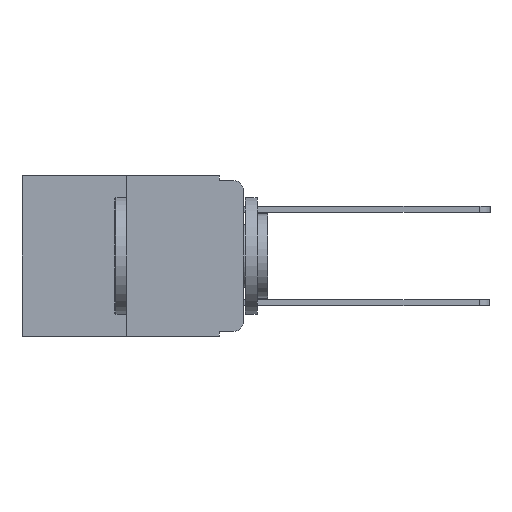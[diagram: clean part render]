
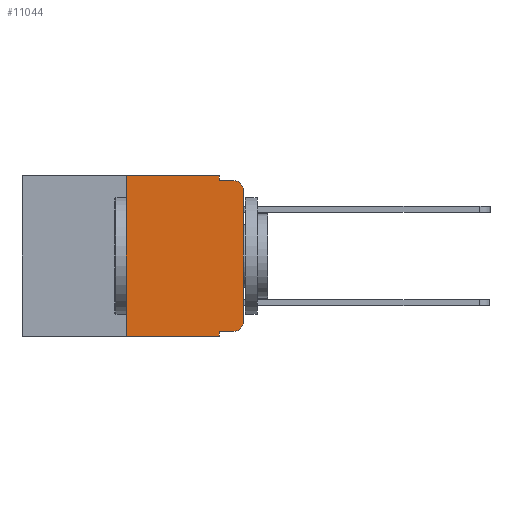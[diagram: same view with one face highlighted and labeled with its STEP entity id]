
A CAD part, left-side view. The second image highlights one B-rep face of the part: STEP entity #11044.
In plain terms, the highlighted planar face has unit normal (-1, 0, 0).
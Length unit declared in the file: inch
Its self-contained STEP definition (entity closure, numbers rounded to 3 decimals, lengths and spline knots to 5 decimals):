
#227 = VERTEX_POINT ( 'NONE', #5715 ) ;
#491 = ORIENTED_EDGE ( 'NONE', *, *, #11624, .F. ) ;
#746 = EDGE_CURVE ( 'NONE', #3006, #7960, #10381, .T. ) ;
#1089 = CARTESIAN_POINT ( 'NONE',  ( 0., 0., 0. ) ) ;
#1142 = VECTOR ( 'NONE', #10765, 39.37008 ) ;
#1330 = VECTOR ( 'NONE', #1624, 39.37008 ) ;
#1410 = CARTESIAN_POINT ( 'NONE',  ( 0., 0.25, -0.343 ) ) ;
#1515 = VECTOR ( 'NONE', #7484, 39.37008 ) ;
#1612 = LINE ( 'NONE', #1089, #14102 ) ;
#1624 = DIRECTION ( 'NONE',  ( 0., 0., -1. ) ) ;
#1700 = LINE ( 'NONE', #18387, #1142 ) ;
#1743 = DIRECTION ( 'NONE',  ( -1., 0., 0. ) ) ;
#2067 = AXIS2_PLACEMENT_3D ( 'NONE', #5316, #17886, #8572 ) ;
#2700 = ORIENTED_EDGE ( 'NONE', *, *, #9438, .T. ) ;
#2933 = DIRECTION ( 'NONE',  ( 0., 0., 1. ) ) ;
#3006 = VERTEX_POINT ( 'NONE', #1410 ) ;
#3287 = VERTEX_POINT ( 'NONE', #15945 ) ;
#3361 = DIRECTION ( 'NONE',  ( 0., -1., 0. ) ) ;
#3600 = CARTESIAN_POINT ( 'NONE',  ( 0., 0.02, -0.03 ) ) ;
#4095 = CARTESIAN_POINT ( 'NONE',  ( 0., 0.051, 0. ) ) ;
#4788 = ORIENTED_EDGE ( 'NONE', *, *, #15676, .T. ) ;
#5189 = CARTESIAN_POINT ( 'NONE',  ( 0., 0.02, -0.01 ) ) ;
#5312 = DIRECTION ( 'NONE',  ( 0., 0., -1. ) ) ;
#5316 = CARTESIAN_POINT ( 'NONE',  ( 0., 0.473, 0. ) ) ;
#5622 = ORIENTED_EDGE ( 'NONE', *, *, #10556, .T. ) ;
#5715 = CARTESIAN_POINT ( 'NONE',  ( 0., 0., -0.03 ) ) ;
#5943 = AXIS2_PLACEMENT_3D ( 'NONE', #3600, #14831, #5312 ) ;
#6291 = CARTESIAN_POINT ( 'NONE',  ( 0., 0.25, 0. ) ) ;
#6614 = CARTESIAN_POINT ( 'NONE',  ( 0., 0.051, 0. ) ) ;
#6912 = PLANE ( 'NONE',  #2067 ) ;
#7179 = CIRCLE ( 'NONE', #16317, 0.02 ) ;
#7484 = DIRECTION ( 'NONE',  ( 0., -1., 0. ) ) ;
#7960 = VERTEX_POINT ( 'NONE', #11419 ) ;
#8572 = DIRECTION ( 'NONE',  ( 0., 0., -1. ) ) ;
#8763 = CARTESIAN_POINT ( 'NONE',  ( 0., 0.02, -0.333 ) ) ;
#9198 = VERTEX_POINT ( 'NONE', #18639 ) ;
#9293 = CARTESIAN_POINT ( 'NONE',  ( 0., 0.051, -0.333 ) ) ;
#9438 = EDGE_CURVE ( 'NONE', #19296, #18883, #7179, .T. ) ;
#10018 = LINE ( 'NONE', #13117, #17720 ) ;
#10020 = EDGE_CURVE ( 'NONE', #3287, #9198, #10018, .T. ) ;
#10178 = ORIENTED_EDGE ( 'NONE', *, *, #14682, .F. ) ;
#10381 = LINE ( 'NONE', #16709, #1515 ) ;
#10556 = EDGE_CURVE ( 'NONE', #10694, #19296, #17216, .T. ) ;
#10694 = VERTEX_POINT ( 'NONE', #9293 ) ;
#10765 = DIRECTION ( 'NONE',  ( 0., -1., 0. ) ) ;
#11044 = ADVANCED_FACE ( 'NONE', ( #12233 ), #6912, .F. ) ;
#11165 = VECTOR ( 'NONE', #15243, 39.37008 ) ;
#11374 = LINE ( 'NONE', #6291, #18998 ) ;
#11419 = CARTESIAN_POINT ( 'NONE',  ( 0., 0.051, -0.343 ) ) ;
#11617 = EDGE_LOOP ( 'NONE', ( #13603, #4788, #10178, #12183, #13861, #17882, #20269, #491, #5622, #2700 ) ) ;
#11624 = EDGE_CURVE ( 'NONE', #10694, #7960, #17895, .T. ) ;
#11640 = CARTESIAN_POINT ( 'NONE',  ( 0., 0.02, -0.313 ) ) ;
#12183 = ORIENTED_EDGE ( 'NONE', *, *, #13694, .F. ) ;
#12233 = FACE_OUTER_BOUND ( 'NONE', #11617, .T. ) ;
#12241 = DIRECTION ( 'NONE',  ( 0., 0., -1. ) ) ;
#12547 = LINE ( 'NONE', #4095, #20148 ) ;
#12654 = EDGE_CURVE ( 'NONE', #3006, #3287, #11374, .T. ) ;
#13117 = CARTESIAN_POINT ( 'NONE',  ( 0., 0.473, 0. ) ) ;
#13208 = DIRECTION ( 'NONE',  ( 0., 0., -1. ) ) ;
#13603 = ORIENTED_EDGE ( 'NONE', *, *, #16724, .T. ) ;
#13694 = EDGE_CURVE ( 'NONE', #9198, #15691, #12547, .T. ) ;
#13861 = ORIENTED_EDGE ( 'NONE', *, *, #10020, .F. ) ;
#14102 = VECTOR ( 'NONE', #17198, 39.37008 ) ;
#14682 = EDGE_CURVE ( 'NONE', #15691, #19795, #1700, .T. ) ;
#14831 = DIRECTION ( 'NONE',  ( -1., 0., 0. ) ) ;
#15181 = CARTESIAN_POINT ( 'NONE',  ( 0., 0.051, -0.333 ) ) ;
#15243 = DIRECTION ( 'NONE',  ( 0., -1., 0. ) ) ;
#15676 = EDGE_CURVE ( 'NONE', #227, #19795, #17186, .T. ) ;
#15691 = VERTEX_POINT ( 'NONE', #16352 ) ;
#15945 = CARTESIAN_POINT ( 'NONE',  ( 0., 0.25, 0. ) ) ;
#16317 = AXIS2_PLACEMENT_3D ( 'NONE', #11640, #1743, #13208 ) ;
#16352 = CARTESIAN_POINT ( 'NONE',  ( 0., 0.051, -0.01 ) ) ;
#16709 = CARTESIAN_POINT ( 'NONE',  ( 0., 0.473, -0.343 ) ) ;
#16724 = EDGE_CURVE ( 'NONE', #18883, #227, #1612, .T. ) ;
#17186 = CIRCLE ( 'NONE', #5943, 0.02 ) ;
#17198 = DIRECTION ( 'NONE',  ( 0., 0., 1. ) ) ;
#17216 = LINE ( 'NONE', #15181, #11165 ) ;
#17720 = VECTOR ( 'NONE', #3361, 39.37008 ) ;
#17882 = ORIENTED_EDGE ( 'NONE', *, *, #12654, .F. ) ;
#17886 = DIRECTION ( 'NONE',  ( 1., 0., 0. ) ) ;
#17895 = LINE ( 'NONE', #6614, #1330 ) ;
#18387 = CARTESIAN_POINT ( 'NONE',  ( 0., 0.051, -0.01 ) ) ;
#18639 = CARTESIAN_POINT ( 'NONE',  ( 0., 0.051, 0. ) ) ;
#18883 = VERTEX_POINT ( 'NONE', #19844 ) ;
#18998 = VECTOR ( 'NONE', #2933, 39.37008 ) ;
#19296 = VERTEX_POINT ( 'NONE', #8763 ) ;
#19795 = VERTEX_POINT ( 'NONE', #5189 ) ;
#19844 = CARTESIAN_POINT ( 'NONE',  ( 0., 0., -0.313 ) ) ;
#20148 = VECTOR ( 'NONE', #12241, 39.37008 ) ;
#20269 = ORIENTED_EDGE ( 'NONE', *, *, #746, .T. ) ;
